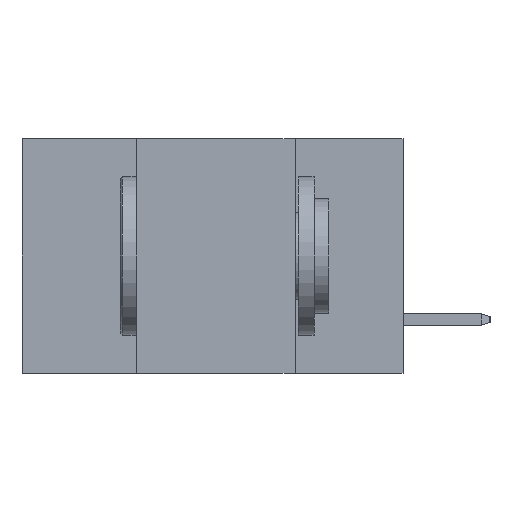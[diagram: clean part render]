
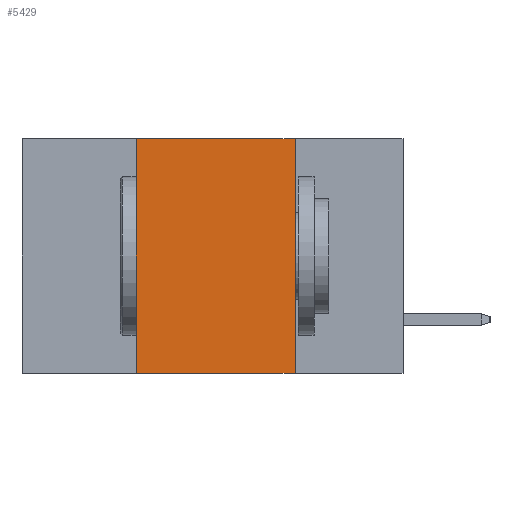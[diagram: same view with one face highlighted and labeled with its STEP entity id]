
A CAD part, left-side view. The second image highlights one B-rep face of the part: STEP entity #5429.
In plain terms, the highlighted planar face has unit normal (-1, 0, 0).
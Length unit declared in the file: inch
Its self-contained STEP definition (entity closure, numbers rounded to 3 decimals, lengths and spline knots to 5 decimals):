
#717 = AXIS2_PLACEMENT_3D ( 'NONE', #10600, #1373, #5842 ) ;
#889 = DIRECTION ( 'NONE',  ( 0., 0., 1. ) ) ;
#1373 = DIRECTION ( 'NONE',  ( 1., 0., 0. ) ) ;
#1870 = VECTOR ( 'NONE', #5509, 39.37008 ) ;
#1922 = LINE ( 'NONE', #4539, #8147 ) ;
#2624 = CARTESIAN_POINT ( 'NONE',  ( 0., 0.6, 0. ) ) ;
#2912 = CARTESIAN_POINT ( 'NONE',  ( 0., 0.42, 0. ) ) ;
#3026 = ORIENTED_EDGE ( 'NONE', *, *, #8726, .F. ) ;
#3061 = EDGE_CURVE ( 'NONE', #10546, #9816, #4334, .T. ) ;
#3988 = FACE_OUTER_BOUND ( 'NONE', #10532, .T. ) ;
#4267 = CARTESIAN_POINT ( 'NONE',  ( 0., 0.42, -0.37 ) ) ;
#4334 = LINE ( 'NONE', #2624, #11230 ) ;
#4408 = LINE ( 'NONE', #10889, #1870 ) ;
#4539 = CARTESIAN_POINT ( 'NONE',  ( 0., 0.42, 0. ) ) ;
#4987 = VECTOR ( 'NONE', #7631, 39.37008 ) ;
#5210 = EDGE_CURVE ( 'NONE', #7203, #10546, #1922, .T. ) ;
#5429 = ADVANCED_FACE ( 'NONE', ( #3988 ), #9757, .F. ) ;
#5509 = DIRECTION ( 'NONE',  ( 0., -1., 0. ) ) ;
#5676 = LINE ( 'NONE', #11108, #4987 ) ;
#5842 = DIRECTION ( 'NONE',  ( 0., 0., -1. ) ) ;
#5907 = ORIENTED_EDGE ( 'NONE', *, *, #3061, .F. ) ;
#6759 = CARTESIAN_POINT ( 'NONE',  ( 0., 0.17, -0.37 ) ) ;
#7203 = VERTEX_POINT ( 'NONE', #4267 ) ;
#7631 = DIRECTION ( 'NONE',  ( 0., 0., -1. ) ) ;
#8106 = EDGE_CURVE ( 'NONE', #7203, #9233, #4408, .T. ) ;
#8147 = VECTOR ( 'NONE', #889, 39.37008 ) ;
#8286 = ORIENTED_EDGE ( 'NONE', *, *, #8106, .T. ) ;
#8654 = CARTESIAN_POINT ( 'NONE',  ( 0., 0.17, 0. ) ) ;
#8726 = EDGE_CURVE ( 'NONE', #9816, #9233, #5676, .T. ) ;
#9216 = ORIENTED_EDGE ( 'NONE', *, *, #5210, .F. ) ;
#9233 = VERTEX_POINT ( 'NONE', #6759 ) ;
#9757 = PLANE ( 'NONE',  #717 ) ;
#9816 = VERTEX_POINT ( 'NONE', #8654 ) ;
#10532 = EDGE_LOOP ( 'NONE', ( #3026, #5907, #9216, #8286 ) ) ;
#10546 = VERTEX_POINT ( 'NONE', #2912 ) ;
#10600 = CARTESIAN_POINT ( 'NONE',  ( 0., 0.6, 0. ) ) ;
#10889 = CARTESIAN_POINT ( 'NONE',  ( 0., 0.6, -0.37 ) ) ;
#11108 = CARTESIAN_POINT ( 'NONE',  ( 0., 0.17, 0. ) ) ;
#11230 = VECTOR ( 'NONE', #11790, 39.37008 ) ;
#11790 = DIRECTION ( 'NONE',  ( 0., -1., 0. ) ) ;
